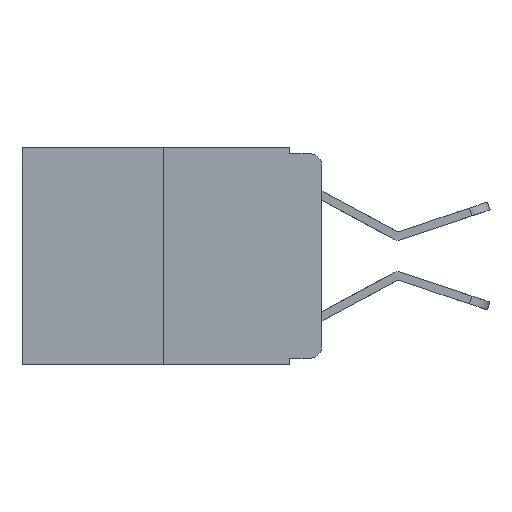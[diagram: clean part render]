
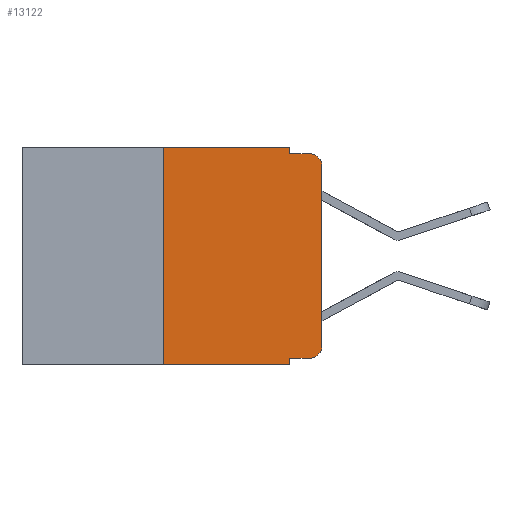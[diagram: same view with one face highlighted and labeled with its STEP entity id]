
A CAD part, left-side view. The second image highlights one B-rep face of the part: STEP entity #13122.
In plain terms, the highlighted planar face has unit normal (-1, 0, 0).
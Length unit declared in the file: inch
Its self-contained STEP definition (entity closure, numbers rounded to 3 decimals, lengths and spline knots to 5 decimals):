
#105 = CARTESIAN_POINT ( 'NONE',  ( 0., 0.25, 0. ) ) ;
#294 = VERTEX_POINT ( 'NONE', #7014 ) ;
#475 = ORIENTED_EDGE ( 'NONE', *, *, #7502, .T. ) ;
#795 = VERTEX_POINT ( 'NONE', #10931 ) ;
#953 = DIRECTION ( 'NONE',  ( 0., 0., -1. ) ) ;
#1060 = VERTEX_POINT ( 'NONE', #11199 ) ;
#1237 = LINE ( 'NONE', #13353, #11879 ) ;
#1324 = ORIENTED_EDGE ( 'NONE', *, *, #5412, .F. ) ;
#1608 = CARTESIAN_POINT ( 'NONE',  ( 0., 0.02, -0.313 ) ) ;
#1635 = ORIENTED_EDGE ( 'NONE', *, *, #2640, .T. ) ;
#1668 = CARTESIAN_POINT ( 'NONE',  ( 0., 0., -0.03 ) ) ;
#1963 = EDGE_LOOP ( 'NONE', ( #7169, #2052, #5900, #10545, #12500, #1324, #1635, #6931, #475, #3441 ) ) ;
#2052 = ORIENTED_EDGE ( 'NONE', *, *, #12823, .T. ) ;
#2640 = EDGE_CURVE ( 'NONE', #9793, #6072, #1237, .T. ) ;
#2719 = DIRECTION ( 'NONE',  ( 0., 0., -1. ) ) ;
#2874 = DIRECTION ( 'NONE',  ( 0., -1., 0. ) ) ;
#2927 = LINE ( 'NONE', #4803, #3274 ) ;
#3028 = EDGE_CURVE ( 'NONE', #294, #10339, #9470, .T. ) ;
#3142 = EDGE_CURVE ( 'NONE', #9589, #6072, #8516, .T. ) ;
#3274 = VECTOR ( 'NONE', #11826, 39.37008 ) ;
#3356 = VECTOR ( 'NONE', #12150, 39.37008 ) ;
#3419 = FACE_OUTER_BOUND ( 'NONE', #1963, .T. ) ;
#3441 = ORIENTED_EDGE ( 'NONE', *, *, #4653, .T. ) ;
#3683 = LINE ( 'NONE', #11177, #3356 ) ;
#3862 = CARTESIAN_POINT ( 'NONE',  ( 0., 0.25, -0.343 ) ) ;
#4314 = CIRCLE ( 'NONE', #5073, 0.02 ) ;
#4401 = DIRECTION ( 'NONE',  ( 0., -1., 0. ) ) ;
#4551 = CARTESIAN_POINT ( 'NONE',  ( 0., 0.051, -0.333 ) ) ;
#4581 = CIRCLE ( 'NONE', #7319, 0.02 ) ;
#4590 = LINE ( 'NONE', #9096, #9715 ) ;
#4626 = DIRECTION ( 'NONE',  ( -1., 0., 0. ) ) ;
#4653 = EDGE_CURVE ( 'NONE', #5470, #11281, #4314, .T. ) ;
#4803 = CARTESIAN_POINT ( 'NONE',  ( 0., 0.473, 0. ) ) ;
#4922 = LINE ( 'NONE', #105, #7343 ) ;
#5073 = AXIS2_PLACEMENT_3D ( 'NONE', #1608, #8949, #2719 ) ;
#5412 = EDGE_CURVE ( 'NONE', #9793, #795, #4922, .T. ) ;
#5456 = VECTOR ( 'NONE', #10267, 39.37008 ) ;
#5470 = VERTEX_POINT ( 'NONE', #5635 ) ;
#5635 = CARTESIAN_POINT ( 'NONE',  ( 0., 0.02, -0.333 ) ) ;
#5900 = ORIENTED_EDGE ( 'NONE', *, *, #12461, .F. ) ;
#6004 = CARTESIAN_POINT ( 'NONE',  ( 0., 0.051, 0. ) ) ;
#6072 = VERTEX_POINT ( 'NONE', #10835 ) ;
#6306 = PLANE ( 'NONE',  #13023 ) ;
#6931 = ORIENTED_EDGE ( 'NONE', *, *, #3142, .F. ) ;
#7014 = CARTESIAN_POINT ( 'NONE',  ( 0., 0.051, 0. ) ) ;
#7024 = VERTEX_POINT ( 'NONE', #1668 ) ;
#7037 = DIRECTION ( 'NONE',  ( 0., 0., -1. ) ) ;
#7169 = ORIENTED_EDGE ( 'NONE', *, *, #7810, .T. ) ;
#7319 = AXIS2_PLACEMENT_3D ( 'NONE', #10718, #4626, #11672 ) ;
#7337 = DIRECTION ( 'NONE',  ( 1., 0., 0. ) ) ;
#7343 = VECTOR ( 'NONE', #8641, 39.37008 ) ;
#7502 = EDGE_CURVE ( 'NONE', #9589, #5470, #9950, .T. ) ;
#7810 = EDGE_CURVE ( 'NONE', #11281, #7024, #3683, .T. ) ;
#8516 = LINE ( 'NONE', #9284, #5456 ) ;
#8641 = DIRECTION ( 'NONE',  ( 0., 0., 1. ) ) ;
#8719 = CARTESIAN_POINT ( 'NONE',  ( 0., 0.051, -0.333 ) ) ;
#8917 = CARTESIAN_POINT ( 'NONE',  ( 0., 0.051, -0.01 ) ) ;
#8949 = DIRECTION ( 'NONE',  ( -1., 0., 0. ) ) ;
#9096 = CARTESIAN_POINT ( 'NONE',  ( 0., 0.051, -0.01 ) ) ;
#9284 = CARTESIAN_POINT ( 'NONE',  ( 0., 0.051, 0. ) ) ;
#9470 = LINE ( 'NONE', #6004, #12053 ) ;
#9589 = VERTEX_POINT ( 'NONE', #4551 ) ;
#9651 = VECTOR ( 'NONE', #11633, 39.37008 ) ;
#9715 = VECTOR ( 'NONE', #2874, 39.37008 ) ;
#9793 = VERTEX_POINT ( 'NONE', #3862 ) ;
#9950 = LINE ( 'NONE', #8719, #9651 ) ;
#10267 = DIRECTION ( 'NONE',  ( 0., 0., -1. ) ) ;
#10316 = EDGE_CURVE ( 'NONE', #795, #294, #2927, .T. ) ;
#10339 = VERTEX_POINT ( 'NONE', #8917 ) ;
#10545 = ORIENTED_EDGE ( 'NONE', *, *, #3028, .F. ) ;
#10718 = CARTESIAN_POINT ( 'NONE',  ( 0., 0.02, -0.03 ) ) ;
#10835 = CARTESIAN_POINT ( 'NONE',  ( 0., 0.051, -0.343 ) ) ;
#10931 = CARTESIAN_POINT ( 'NONE',  ( 0., 0.25, 0. ) ) ;
#11177 = CARTESIAN_POINT ( 'NONE',  ( 0., 0., 0. ) ) ;
#11199 = CARTESIAN_POINT ( 'NONE',  ( 0., 0.02, -0.01 ) ) ;
#11281 = VERTEX_POINT ( 'NONE', #11635 ) ;
#11633 = DIRECTION ( 'NONE',  ( 0., -1., 0. ) ) ;
#11635 = CARTESIAN_POINT ( 'NONE',  ( 0., 0., -0.313 ) ) ;
#11672 = DIRECTION ( 'NONE',  ( 0., 0., -1. ) ) ;
#11826 = DIRECTION ( 'NONE',  ( 0., -1., 0. ) ) ;
#11879 = VECTOR ( 'NONE', #4401, 39.37008 ) ;
#12053 = VECTOR ( 'NONE', #7037, 39.37008 ) ;
#12150 = DIRECTION ( 'NONE',  ( 0., 0., 1. ) ) ;
#12461 = EDGE_CURVE ( 'NONE', #10339, #1060, #4590, .T. ) ;
#12500 = ORIENTED_EDGE ( 'NONE', *, *, #10316, .F. ) ;
#12823 = EDGE_CURVE ( 'NONE', #7024, #1060, #4581, .T. ) ;
#13023 = AXIS2_PLACEMENT_3D ( 'NONE', #13204, #7337, #953 ) ;
#13122 = ADVANCED_FACE ( 'NONE', ( #3419 ), #6306, .F. ) ;
#13204 = CARTESIAN_POINT ( 'NONE',  ( 0., 0.473, 0. ) ) ;
#13353 = CARTESIAN_POINT ( 'NONE',  ( 0., 0.473, -0.343 ) ) ;
